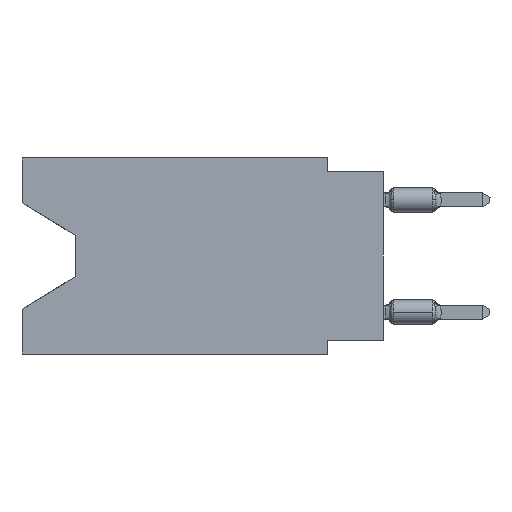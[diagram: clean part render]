
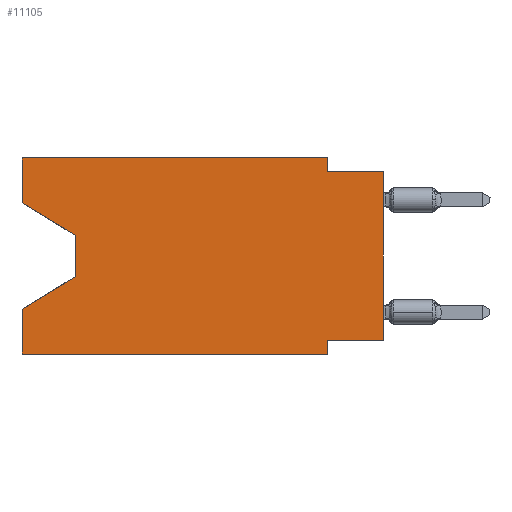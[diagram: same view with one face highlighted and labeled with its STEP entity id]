
A CAD part, left-side view. The second image highlights one B-rep face of the part: STEP entity #11105.
In plain terms, the highlighted planar face has unit normal (-1, 0, 0).
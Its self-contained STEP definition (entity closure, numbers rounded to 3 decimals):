
#17 = VERTEX_POINT ( 'NONE', #52564 ) ;
#158 = VERTEX_POINT ( 'NONE', #44071 ) ;
#308 = LINE ( 'NONE', #42134, #30325 ) ;
#622 = DIRECTION ( 'NONE',  ( 0., 0., 1. ) ) ;
#785 = VECTOR ( 'NONE', #20405, 1000. ) ;
#804 = DIRECTION ( 'NONE',  ( 0., 0., 1. ) ) ;
#1021 = DIRECTION ( 'NONE',  ( 0., -1., 0. ) ) ;
#1160 = CARTESIAN_POINT ( 'NONE',  ( 0., 13.97, -5.385 ) ) ;
#2286 = VERTEX_POINT ( 'NONE', #22687 ) ;
#2681 = EDGE_CURVE ( 'NONE', #47488, #4969, #14354, .T. ) ;
#2896 = VECTOR ( 'NONE', #51634, 1000. ) ;
#2963 = VERTEX_POINT ( 'NONE', #44619 ) ;
#2987 = VECTOR ( 'NONE', #1021, 1000. ) ;
#4969 = VERTEX_POINT ( 'NONE', #22506 ) ;
#6469 = LINE ( 'NONE', #11302, #785 ) ;
#7076 = EDGE_CURVE ( 'NONE', #4969, #39438, #37842, .T. ) ;
#8415 = CARTESIAN_POINT ( 'NONE',  ( 0., 2.54, 0. ) ) ;
#8467 = ORIENTED_EDGE ( 'NONE', *, *, #42658, .T. ) ;
#10236 = DIRECTION ( 'NONE',  ( 0., 0.855, -0.519 ) ) ;
#11105 = ADVANCED_FACE ( 'NONE', ( #36097 ), #50030, .F. ) ;
#11258 = VERTEX_POINT ( 'NONE', #28234 ) ;
#11302 = CARTESIAN_POINT ( 'NONE',  ( 0., 16.383, 0. ) ) ;
#12786 = VERTEX_POINT ( 'NONE', #25863 ) ;
#13379 = ORIENTED_EDGE ( 'NONE', *, *, #2681, .T. ) ;
#13532 = ORIENTED_EDGE ( 'NONE', *, *, #24901, .F. ) ;
#13659 = DIRECTION ( 'NONE',  ( 0., 0., -1. ) ) ;
#13794 = ORIENTED_EDGE ( 'NONE', *, *, #7076, .T. ) ;
#14065 = CARTESIAN_POINT ( 'NONE',  ( 0., 2.54, -8.89 ) ) ;
#14354 = LINE ( 'NONE', #23455, #2896 ) ;
#18974 = CARTESIAN_POINT ( 'NONE',  ( 0., 16.383, 0. ) ) ;
#20315 = LINE ( 'NONE', #57006, #32567 ) ;
#20405 = DIRECTION ( 'NONE',  ( 0., -1., 0. ) ) ;
#21748 = EDGE_LOOP ( 'NONE', ( #56001, #13379, #13794, #30094, #48930, #59813, #29390, #8467, #46723, #36267, #57615, #13532 ) ) ;
#22005 = CARTESIAN_POINT ( 'NONE',  ( 0., 0., -8.255 ) ) ;
#22449 = CARTESIAN_POINT ( 'NONE',  ( 0., 16.383, 0. ) ) ;
#22506 = CARTESIAN_POINT ( 'NONE',  ( 0., 13.97, -5.385 ) ) ;
#22687 = CARTESIAN_POINT ( 'NONE',  ( 0., 2.54, -8.255 ) ) ;
#22719 = CARTESIAN_POINT ( 'NONE',  ( 0., 16.383, -2.038 ) ) ;
#22911 = LINE ( 'NONE', #22005, #43685 ) ;
#23455 = CARTESIAN_POINT ( 'NONE',  ( 0., 13.97, -3.505 ) ) ;
#23830 = LINE ( 'NONE', #18974, #45386 ) ;
#24072 = LINE ( 'NONE', #33176, #42362 ) ;
#24901 = EDGE_CURVE ( 'NONE', #57096, #11258, #23830, .T. ) ;
#24952 = CARTESIAN_POINT ( 'NONE',  ( 0., 16.383, -6.852 ) ) ;
#25863 = CARTESIAN_POINT ( 'NONE',  ( 0., 0., -0.635 ) ) ;
#26077 = DIRECTION ( 'NONE',  ( 0., -0.855, -0.519 ) ) ;
#27003 = CARTESIAN_POINT ( 'NONE',  ( 0., 13.97, -3.505 ) ) ;
#28234 = CARTESIAN_POINT ( 'NONE',  ( 0., 16.383, 0. ) ) ;
#28294 = VECTOR ( 'NONE', #54807, 1000. ) ;
#29390 = ORIENTED_EDGE ( 'NONE', *, *, #35497, .F. ) ;
#30069 = EDGE_CURVE ( 'NONE', #2286, #49991, #24072, .T. ) ;
#30094 = ORIENTED_EDGE ( 'NONE', *, *, #54875, .F. ) ;
#30325 = VECTOR ( 'NONE', #622, 1000. ) ;
#32567 = VECTOR ( 'NONE', #42776, 1000. ) ;
#33176 = CARTESIAN_POINT ( 'NONE',  ( 0., 2.54, -8.89 ) ) ;
#33435 = LINE ( 'NONE', #42533, #2987 ) ;
#34529 = AXIS2_PLACEMENT_3D ( 'NONE', #22449, #54881, #13659 ) ;
#35497 = EDGE_CURVE ( 'NONE', #17, #2286, #22911, .T. ) ;
#35605 = LINE ( 'NONE', #54387, #41309 ) ;
#36097 = FACE_OUTER_BOUND ( 'NONE', #21748, .T. ) ;
#36249 = DIRECTION ( 'NONE',  ( 0., 1., 0. ) ) ;
#36267 = ORIENTED_EDGE ( 'NONE', *, *, #56400, .F. ) ;
#37730 = DIRECTION ( 'NONE',  ( 0., 0., -1. ) ) ;
#37842 = LINE ( 'NONE', #1160, #43083 ) ;
#38467 = EDGE_CURVE ( 'NONE', #11258, #42943, #6469, .T. ) ;
#39438 = VERTEX_POINT ( 'NONE', #24952 ) ;
#41018 = VECTOR ( 'NONE', #26077, 1000. ) ;
#41199 = EDGE_CURVE ( 'NONE', #57096, #47488, #54256, .T. ) ;
#41309 = VECTOR ( 'NONE', #54075, 1000. ) ;
#42134 = CARTESIAN_POINT ( 'NONE',  ( 0., 0., 0. ) ) ;
#42362 = VECTOR ( 'NONE', #37730, 1000. ) ;
#42533 = CARTESIAN_POINT ( 'NONE',  ( 0., 16.383, -8.89 ) ) ;
#42658 = EDGE_CURVE ( 'NONE', #17, #12786, #308, .T. ) ;
#42776 = DIRECTION ( 'NONE',  ( 0., 0., -1. ) ) ;
#42943 = VERTEX_POINT ( 'NONE', #8415 ) ;
#43083 = VECTOR ( 'NONE', #10236, 1000. ) ;
#43685 = VECTOR ( 'NONE', #36249, 1000. ) ;
#44071 = CARTESIAN_POINT ( 'NONE',  ( 0., 16.383, -8.89 ) ) ;
#44619 = CARTESIAN_POINT ( 'NONE',  ( 0., 2.54, -0.635 ) ) ;
#44798 = EDGE_CURVE ( 'NONE', #158, #49991, #33435, .T. ) ;
#45386 = VECTOR ( 'NONE', #804, 1000. ) ;
#45481 = EDGE_CURVE ( 'NONE', #2963, #12786, #49958, .T. ) ;
#46723 = ORIENTED_EDGE ( 'NONE', *, *, #45481, .F. ) ;
#47488 = VERTEX_POINT ( 'NONE', #27003 ) ;
#48930 = ORIENTED_EDGE ( 'NONE', *, *, #44798, .T. ) ;
#49958 = LINE ( 'NONE', #59660, #28294 ) ;
#49991 = VERTEX_POINT ( 'NONE', #14065 ) ;
#50030 = PLANE ( 'NONE',  #34529 ) ;
#51634 = DIRECTION ( 'NONE',  ( 0., 0., -1. ) ) ;
#52564 = CARTESIAN_POINT ( 'NONE',  ( 0., 0., -8.255 ) ) ;
#54075 = DIRECTION ( 'NONE',  ( 0., 0., 1. ) ) ;
#54256 = LINE ( 'NONE', #22719, #41018 ) ;
#54387 = CARTESIAN_POINT ( 'NONE',  ( 0., 16.383, 0. ) ) ;
#54682 = CARTESIAN_POINT ( 'NONE',  ( 0., 16.383, -2.038 ) ) ;
#54807 = DIRECTION ( 'NONE',  ( 0., -1., 0. ) ) ;
#54875 = EDGE_CURVE ( 'NONE', #158, #39438, #35605, .T. ) ;
#54881 = DIRECTION ( 'NONE',  ( 1., 0., 0. ) ) ;
#56001 = ORIENTED_EDGE ( 'NONE', *, *, #41199, .T. ) ;
#56400 = EDGE_CURVE ( 'NONE', #42943, #2963, #20315, .T. ) ;
#57006 = CARTESIAN_POINT ( 'NONE',  ( 0., 2.54, 0. ) ) ;
#57096 = VERTEX_POINT ( 'NONE', #54682 ) ;
#57615 = ORIENTED_EDGE ( 'NONE', *, *, #38467, .F. ) ;
#59660 = CARTESIAN_POINT ( 'NONE',  ( 0., 0., -0.635 ) ) ;
#59813 = ORIENTED_EDGE ( 'NONE', *, *, #30069, .F. ) ;
